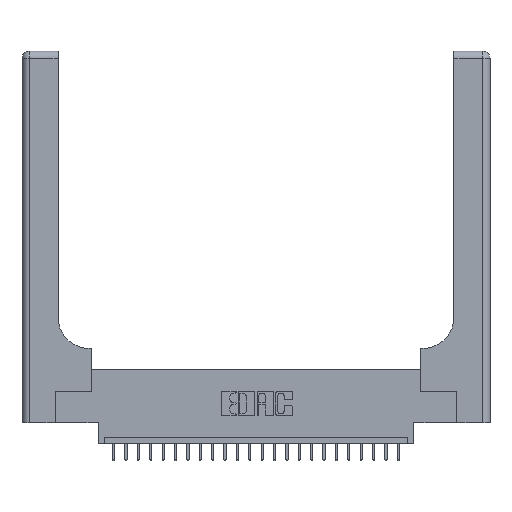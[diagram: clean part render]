
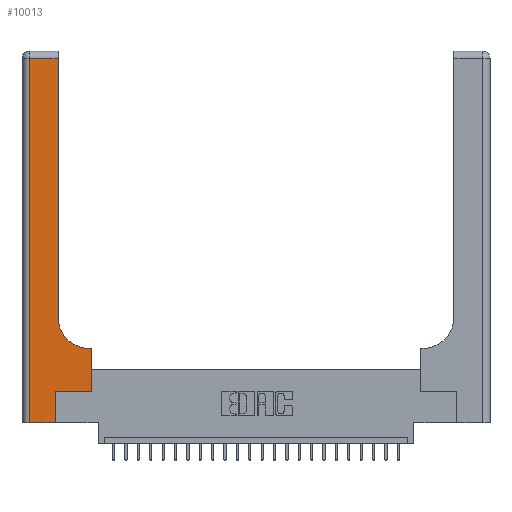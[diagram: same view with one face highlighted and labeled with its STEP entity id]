
A CAD part, top view. The second image highlights one B-rep face of the part: STEP entity #10013.
In plain terms, the highlighted planar face has unit normal (0, 0, 1).
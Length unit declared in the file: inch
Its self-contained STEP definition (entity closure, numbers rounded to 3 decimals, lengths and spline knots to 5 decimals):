
#192 = ORIENTED_EDGE ( 'NONE', *, *, #2626, .T. ) ;
#384 = ORIENTED_EDGE ( 'NONE', *, *, #15084, .T. ) ;
#576 = DIRECTION ( 'NONE',  ( -1., 0., 0. ) ) ;
#634 = FACE_OUTER_BOUND ( 'NONE', #8541, .T. ) ;
#1505 = CARTESIAN_POINT ( 'NONE',  ( 0.2915, 3., 0.37 ) ) ;
#1704 = VERTEX_POINT ( 'NONE', #12048 ) ;
#1857 = CARTESIAN_POINT ( 'NONE',  ( 0., 0., 0.37 ) ) ;
#2256 = EDGE_CURVE ( 'NONE', #7489, #20517, #12769, .T. ) ;
#2626 = EDGE_CURVE ( 'NONE', #20517, #11758, #16673, .T. ) ;
#2829 = VECTOR ( 'NONE', #23771, 39.37008 ) ;
#2850 = EDGE_CURVE ( 'NONE', #13948, #11046, #17436, .T. ) ;
#3391 = ORIENTED_EDGE ( 'NONE', *, *, #2850, .T. ) ;
#3704 = CARTESIAN_POINT ( 'NONE',  ( 0.269, 0., 0.37 ) ) ;
#3903 = CARTESIAN_POINT ( 'NONE',  ( 0.269, 0., 0.37 ) ) ;
#4156 = ORIENTED_EDGE ( 'NONE', *, *, #24766, .T. ) ;
#4319 = DIRECTION ( 'NONE',  ( 0., 0., -1. ) ) ;
#4357 = CARTESIAN_POINT ( 'NONE',  ( 0.5585, 0.25, 0.37 ) ) ;
#4661 = VECTOR ( 'NONE', #18637, 39.37008 ) ;
#4664 = DIRECTION ( 'NONE',  ( 0., 1., 0. ) ) ;
#5359 = ORIENTED_EDGE ( 'NONE', *, *, #21966, .T. ) ;
#5794 = LINE ( 'NONE', #1857, #6157 ) ;
#5852 = VECTOR ( 'NONE', #11705, 39.37008 ) ;
#5970 = VECTOR ( 'NONE', #4664, 39.37008 ) ;
#6157 = VECTOR ( 'NONE', #6333, 39.37008 ) ;
#6333 = DIRECTION ( 'NONE',  ( 1., 0., 0. ) ) ;
#7489 = VERTEX_POINT ( 'NONE', #4357 ) ;
#7495 = DIRECTION ( 'NONE',  ( -1., 0., 0. ) ) ;
#7720 = EDGE_CURVE ( 'NONE', #25611, #7489, #10884, .T. ) ;
#7992 = ORIENTED_EDGE ( 'NONE', *, *, #7720, .T. ) ;
#8230 = CARTESIAN_POINT ( 'NONE',  ( 0.269, 0.25, 0.37 ) ) ;
#8541 = EDGE_LOOP ( 'NONE', ( #5359, #3391, #384, #13010, #10079, #7992, #17327, #192, #4156 ) ) ;
#8766 = PLANE ( 'NONE',  #12900 ) ;
#9192 = CIRCLE ( 'NONE', #23824, 0.25 ) ;
#10013 = ADVANCED_FACE ( 'NONE', ( #634 ), #8766, .F. ) ;
#10079 = ORIENTED_EDGE ( 'NONE', *, *, #13656, .T. ) ;
#10884 = LINE ( 'NONE', #20725, #22032 ) ;
#11046 = VERTEX_POINT ( 'NONE', #13262 ) ;
#11411 = CARTESIAN_POINT ( 'NONE',  ( 0.06, 0., 0.37 ) ) ;
#11705 = DIRECTION ( 'NONE',  ( 0., 1., 0. ) ) ;
#11758 = VERTEX_POINT ( 'NONE', #17341 ) ;
#12048 = CARTESIAN_POINT ( 'NONE',  ( 0.2915, 0.85, 0.37 ) ) ;
#12129 = DIRECTION ( 'NONE',  ( 1., 0., 0. ) ) ;
#12769 = LINE ( 'NONE', #16319, #5970 ) ;
#12807 = CARTESIAN_POINT ( 'NONE',  ( 0., 3., 0.37 ) ) ;
#12900 = AXIS2_PLACEMENT_3D ( 'NONE', #12807, #4319, #20285 ) ;
#13010 = ORIENTED_EDGE ( 'NONE', *, *, #20716, .T. ) ;
#13262 = CARTESIAN_POINT ( 'NONE',  ( 0.06, 2.94, 0.37 ) ) ;
#13656 = EDGE_CURVE ( 'NONE', #16668, #25611, #21657, .T. ) ;
#13779 = CARTESIAN_POINT ( 'NONE',  ( 0., 2.94, 0.37 ) ) ;
#13948 = VERTEX_POINT ( 'NONE', #21242 ) ;
#15084 = EDGE_CURVE ( 'NONE', #11046, #24993, #24906, .T. ) ;
#16319 = CARTESIAN_POINT ( 'NONE',  ( 0.5585, 0.25, 0.37 ) ) ;
#16668 = VERTEX_POINT ( 'NONE', #3903 ) ;
#16673 = LINE ( 'NONE', #22323, #25210 ) ;
#16860 = VECTOR ( 'NONE', #7495, 39.37008 ) ;
#17064 = CARTESIAN_POINT ( 'NONE',  ( 0.5585, 0.6, 0.37 ) ) ;
#17327 = ORIENTED_EDGE ( 'NONE', *, *, #2256, .T. ) ;
#17341 = CARTESIAN_POINT ( 'NONE',  ( 0.5415, 0.6, 0.37 ) ) ;
#17436 = LINE ( 'NONE', #13779, #16860 ) ;
#18637 = DIRECTION ( 'NONE',  ( 0., -1., 0. ) ) ;
#19975 = CARTESIAN_POINT ( 'NONE',  ( 0.5415, 0.85, 0.37 ) ) ;
#20285 = DIRECTION ( 'NONE',  ( -1., 0., 0. ) ) ;
#20517 = VERTEX_POINT ( 'NONE', #17064 ) ;
#20716 = EDGE_CURVE ( 'NONE', #24993, #16668, #5794, .T. ) ;
#20725 = CARTESIAN_POINT ( 'NONE',  ( 0.269, 0.25, 0.37 ) ) ;
#21242 = CARTESIAN_POINT ( 'NONE',  ( 0.2915, 2.94, 0.37 ) ) ;
#21657 = LINE ( 'NONE', #3704, #5852 ) ;
#21966 = EDGE_CURVE ( 'NONE', #1704, #13948, #25742, .T. ) ;
#22032 = VECTOR ( 'NONE', #22801, 39.37008 ) ;
#22323 = CARTESIAN_POINT ( 'NONE',  ( 0.2915, 0.6, 0.37 ) ) ;
#22706 = CARTESIAN_POINT ( 'NONE',  ( 0.06, 3., 0.37 ) ) ;
#22801 = DIRECTION ( 'NONE',  ( 1., 0., 0. ) ) ;
#23766 = DIRECTION ( 'NONE',  ( 0., 0., -1. ) ) ;
#23771 = DIRECTION ( 'NONE',  ( 0., 1., 0. ) ) ;
#23824 = AXIS2_PLACEMENT_3D ( 'NONE', #19975, #23766, #12129 ) ;
#24766 = EDGE_CURVE ( 'NONE', #11758, #1704, #9192, .T. ) ;
#24906 = LINE ( 'NONE', #22706, #4661 ) ;
#24993 = VERTEX_POINT ( 'NONE', #11411 ) ;
#25210 = VECTOR ( 'NONE', #576, 39.37008 ) ;
#25611 = VERTEX_POINT ( 'NONE', #8230 ) ;
#25742 = LINE ( 'NONE', #1505, #2829 ) ;
